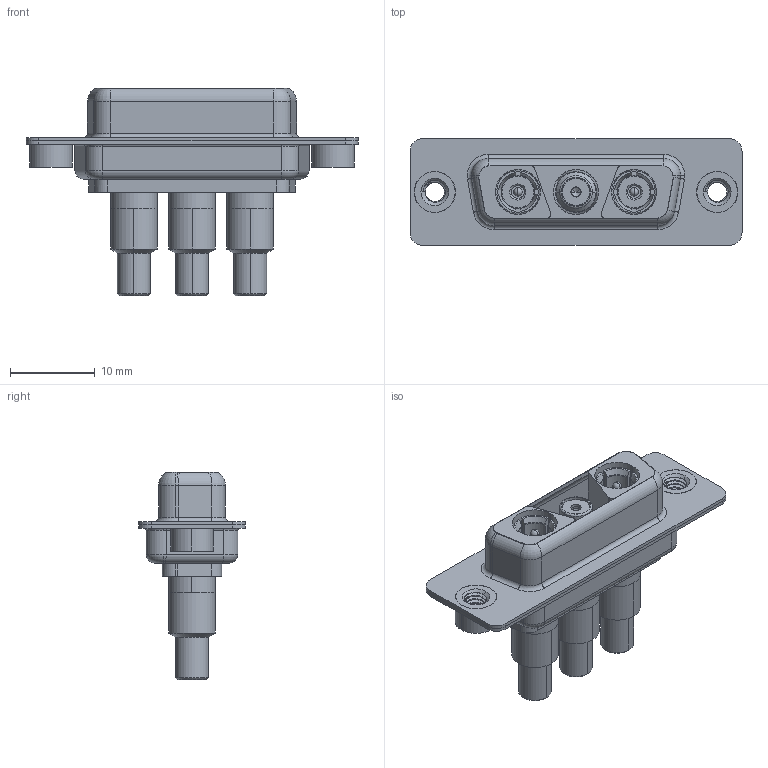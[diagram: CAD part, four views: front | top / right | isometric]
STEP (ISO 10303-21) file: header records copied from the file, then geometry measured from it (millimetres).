
FILE_DESCRIPTION (( 'STEP AP203' ), '1' );
FILE_NAME ('628-3WK3222-7TA.STEP', '2019-05-29T07:12:52', ( '' ), ( '' ), 'SwSTEP 2.0', 'SolidWorks 2016', '' );
FILE_SCHEMA (( 'CONFIG_CONTROL_DESIGN' ));
Length unit declared in the file: millimetre
Products named in the file (16): Socket_Solder Cup; Insulator Pin_Solder Cup Tail; Co-Ax Jack Assy_SC; Pin_Solder Cup; 628-3WK3222-7TA; Locking Collar; Solder Cover; 628Combo Housing_3WK3; Co-Ax Plug Assy_SC; 628Combo Shell Front_15 Contacts; Co-Ax Jack_Solder Cup Tail; 628Combo Shell Rear_15 Contacts; Insulator Socket; 628Combo Threaded Rivet_A; Insulator Socket 2; Co-Ax Plug_Solder Cup Tail
Assembly tree (19 placements, depth 3):
  628-3WK3222-7TA
    628Combo Housing_3WK3
    628Combo Shell Front_15 Contacts
    628Combo Shell Rear_15 Contacts
    628Combo Threaded Rivet_A  x2
    Co-Ax Plug Assy_SC  x2
      Co-Ax Plug_Solder Cup Tail
      Insulator Pin_Solder Cup Tail
      Pin_Solder Cup
      Locking Collar
      Solder Cover
    Co-Ax Jack Assy_SC
      Co-Ax Jack_Solder Cup Tail
      Insulator Socket
      Insulator Socket 2
      Locking Collar
      Socket_Solder Cup
      Solder Cover
Bounding box: 39.15 x 12.6 x 24.45 mm (x, y, z)
Volume: 2550.5 mm3; surface area: 7576.6 mm2
Topology: 21 solids, 21 shells, 709 faces, 1685 edges, 1045 vertices
Faces by surface type: cylinder 332, plane 212, cone 80, torus 69, bspline 12, sphere 4
Entity records: 18689 total; most frequent: CARTESIAN_POINT 4751, DIRECTION 2743, ORIENTED_EDGE 2418, EDGE_CURVE 1209, AXIS2_PLACEMENT_3D 1113, VERTEX_POINT 757, CIRCLE 583, EDGE_LOOP 580
